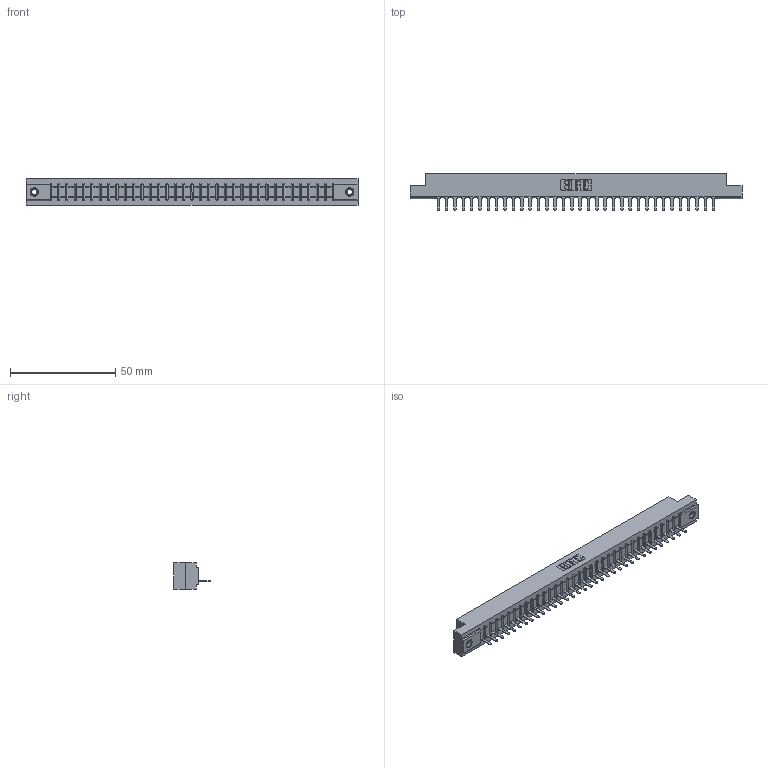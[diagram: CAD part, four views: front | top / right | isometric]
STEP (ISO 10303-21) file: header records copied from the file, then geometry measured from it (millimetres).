
FILE_DESCRIPTION (( 'STEP AP203' ), '1' );
FILE_NAME ('307-034-525-107.STEP', '2019-09-04T02:13:23', ( '' ), ( '' ), 'SwSTEP 2.0', 'SolidWorks 2016', '' );
FILE_SCHEMA (( 'CONFIG_CONTROL_DESIGN' ));
Length unit declared in the file: inch
Products named in the file (4): 307-290-001_525; 307 Part_.156 Dia Mounting Holes; 307-034-525-107; 345-250-001_345-250-005-103
Assembly tree (37 placements, depth 2):
  307-034-525-107
    307 Part_.156 Dia Mounting Holes
    307-290-001_525  x34
    345-250-001_345-250-005-103  x2
Bounding box: 157.73 x 17.42 x 12.7 mm (x, y, z)
Volume: 16289.2 mm3; surface area: 16977.4 mm2
Topology: 37 solids, 37 shells, 2117 faces, 5967 edges, 3830 vertices
Faces by surface type: plane 1360, cylinder 671, sphere 70, cone 12, torus 4
Entity records: 31287 total; most frequent: CARTESIAN_POINT 5247, ORIENTED_EDGE 5226, DIRECTION 5117, EDGE_CURVE 2613, LINE 2001, VECTOR 2001, VERTEX_POINT 1688, AXIS2_PLACEMENT_3D 1558
